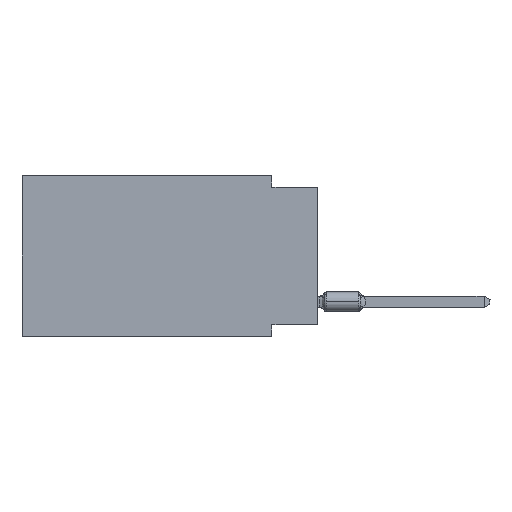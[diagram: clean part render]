
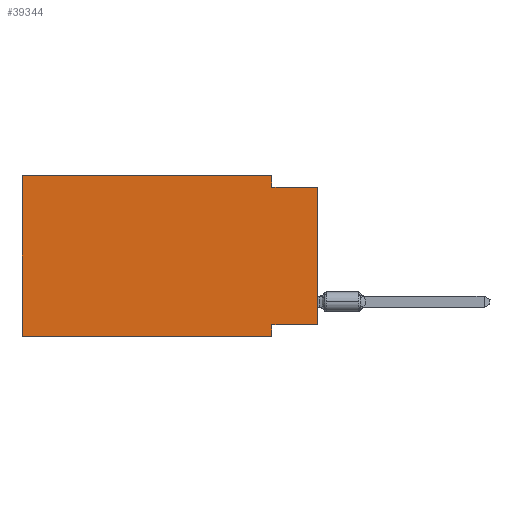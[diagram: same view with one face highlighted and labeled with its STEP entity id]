
A CAD part, left-side view. The second image highlights one B-rep face of the part: STEP entity #39344.
In plain terms, the highlighted planar face has unit normal (-1, 0, 0).
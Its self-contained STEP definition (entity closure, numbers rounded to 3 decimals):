
#15 = EDGE_CURVE ( 'NONE', #61451, #27090, #44090, .T. ) ;
#716 = CARTESIAN_POINT ( 'NONE',  ( 0., 16.383, 0. ) ) ;
#1193 = VECTOR ( 'NONE', #7951, 1000. ) ;
#1765 = CARTESIAN_POINT ( 'NONE',  ( 0., 2.54, 0. ) ) ;
#2472 = CARTESIAN_POINT ( 'NONE',  ( 0., 2.54, -8.89 ) ) ;
#2806 = DIRECTION ( 'NONE',  ( 0., 0., -1. ) ) ;
#3802 = CARTESIAN_POINT ( 'NONE',  ( 0., 2.54, -0.635 ) ) ;
#4014 = DIRECTION ( 'NONE',  ( 0., 0., -1. ) ) ;
#4303 = CARTESIAN_POINT ( 'NONE',  ( 0., 16.383, 0. ) ) ;
#4475 = DIRECTION ( 'NONE',  ( 0., -1., 0. ) ) ;
#6273 = ORIENTED_EDGE ( 'NONE', *, *, #61973, .F. ) ;
#7951 = DIRECTION ( 'NONE',  ( 0., 0., 1. ) ) ;
#9483 = VECTOR ( 'NONE', #2806, 1000. ) ;
#11450 = VECTOR ( 'NONE', #4475, 1000. ) ;
#11534 = CARTESIAN_POINT ( 'NONE',  ( 0., 2.54, -8.255 ) ) ;
#12977 = VECTOR ( 'NONE', #33234, 1000. ) ;
#13128 = CARTESIAN_POINT ( 'NONE',  ( 0., 2.54, -8.89 ) ) ;
#13956 = EDGE_CURVE ( 'NONE', #35191, #37218, #50435, .T. ) ;
#14851 = FACE_OUTER_BOUND ( 'NONE', #62957, .T. ) ;
#14859 = ORIENTED_EDGE ( 'NONE', *, *, #49405, .F. ) ;
#17365 = CARTESIAN_POINT ( 'NONE',  ( 0., 0., -0.635 ) ) ;
#18925 = CARTESIAN_POINT ( 'NONE',  ( 0., 16.383, -8.89 ) ) ;
#20708 = VERTEX_POINT ( 'NONE', #1765 ) ;
#21596 = VECTOR ( 'NONE', #22675, 1000. ) ;
#22675 = DIRECTION ( 'NONE',  ( 0., -1., 0. ) ) ;
#22973 = LINE ( 'NONE', #31625, #53019 ) ;
#24159 = PLANE ( 'NONE',  #32666 ) ;
#27090 = VERTEX_POINT ( 'NONE', #716 ) ;
#27468 = DIRECTION ( 'NONE',  ( 0., 0., -1. ) ) ;
#27487 = LINE ( 'NONE', #46993, #21596 ) ;
#27823 = ORIENTED_EDGE ( 'NONE', *, *, #36385, .F. ) ;
#29572 = DIRECTION ( 'NONE',  ( 0., -1., 0. ) ) ;
#29806 = VERTEX_POINT ( 'NONE', #13128 ) ;
#30214 = EDGE_CURVE ( 'NONE', #35191, #44816, #41550, .T. ) ;
#30217 = EDGE_CURVE ( 'NONE', #61451, #29806, #27487, .T. ) ;
#31625 = CARTESIAN_POINT ( 'NONE',  ( 0., 2.54, 0. ) ) ;
#32619 = EDGE_CURVE ( 'NONE', #44164, #44816, #39667, .T. ) ;
#32666 = AXIS2_PLACEMENT_3D ( 'NONE', #49099, #48793, #4014 ) ;
#33234 = DIRECTION ( 'NONE',  ( 0., 0., 1. ) ) ;
#34002 = ORIENTED_EDGE ( 'NONE', *, *, #32619, .F. ) ;
#35191 = VERTEX_POINT ( 'NONE', #56984 ) ;
#36024 = CARTESIAN_POINT ( 'NONE',  ( 0., 0., -8.255 ) ) ;
#36385 = EDGE_CURVE ( 'NONE', #37218, #29806, #46641, .T. ) ;
#37218 = VERTEX_POINT ( 'NONE', #11534 ) ;
#37382 = CARTESIAN_POINT ( 'NONE',  ( 0., 0., 0. ) ) ;
#37622 = ORIENTED_EDGE ( 'NONE', *, *, #15, .F. ) ;
#39344 = ADVANCED_FACE ( 'NONE', ( #14851 ), #24159, .F. ) ;
#39351 = CARTESIAN_POINT ( 'NONE',  ( 0., 0., -0.635 ) ) ;
#39667 = LINE ( 'NONE', #39351, #11450 ) ;
#41550 = LINE ( 'NONE', #37382, #1193 ) ;
#42761 = VECTOR ( 'NONE', #29572, 1000. ) ;
#44090 = LINE ( 'NONE', #57569, #12977 ) ;
#44164 = VERTEX_POINT ( 'NONE', #3802 ) ;
#44816 = VERTEX_POINT ( 'NONE', #17365 ) ;
#46641 = LINE ( 'NONE', #2472, #9483 ) ;
#46993 = CARTESIAN_POINT ( 'NONE',  ( 0., 16.383, -8.89 ) ) ;
#48456 = LINE ( 'NONE', #4303, #42761 ) ;
#48649 = ORIENTED_EDGE ( 'NONE', *, *, #13956, .F. ) ;
#48793 = DIRECTION ( 'NONE',  ( 1., 0., 0. ) ) ;
#49099 = CARTESIAN_POINT ( 'NONE',  ( 0., 16.383, 0. ) ) ;
#49405 = EDGE_CURVE ( 'NONE', #27090, #20708, #48456, .T. ) ;
#50435 = LINE ( 'NONE', #36024, #53586 ) ;
#53019 = VECTOR ( 'NONE', #27468, 1000. ) ;
#53586 = VECTOR ( 'NONE', #61944, 1000. ) ;
#56051 = ORIENTED_EDGE ( 'NONE', *, *, #30217, .T. ) ;
#56984 = CARTESIAN_POINT ( 'NONE',  ( 0., 0., -8.255 ) ) ;
#57569 = CARTESIAN_POINT ( 'NONE',  ( 0., 16.383, 0. ) ) ;
#58994 = ORIENTED_EDGE ( 'NONE', *, *, #30214, .T. ) ;
#61451 = VERTEX_POINT ( 'NONE', #18925 ) ;
#61944 = DIRECTION ( 'NONE',  ( 0., 1., 0. ) ) ;
#61973 = EDGE_CURVE ( 'NONE', #20708, #44164, #22973, .T. ) ;
#62957 = EDGE_LOOP ( 'NONE', ( #58994, #34002, #6273, #14859, #37622, #56051, #27823, #48649 ) ) ;
